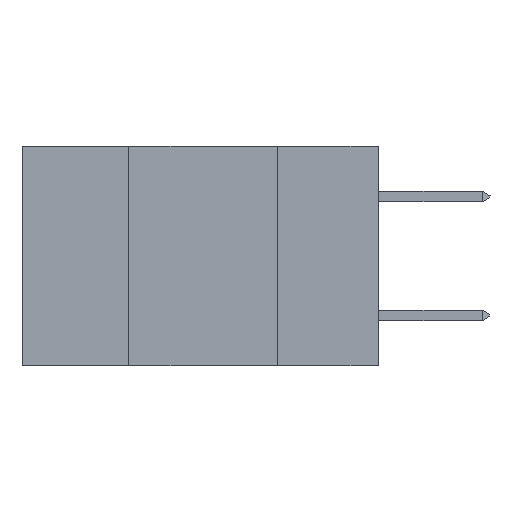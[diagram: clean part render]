
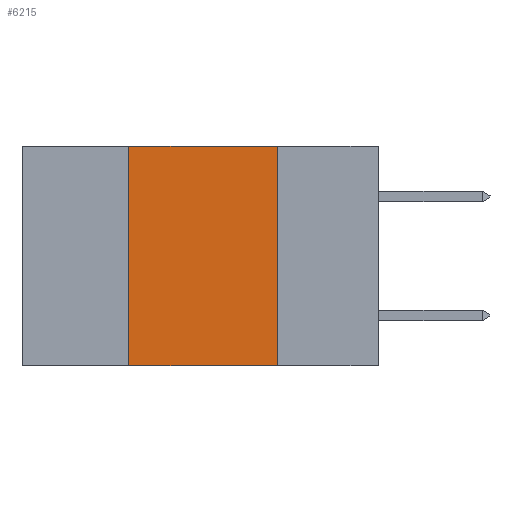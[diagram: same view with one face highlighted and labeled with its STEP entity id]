
A CAD part, left-side view. The second image highlights one B-rep face of the part: STEP entity #6215.
In plain terms, the highlighted planar face has unit normal (-1, 0, 0).
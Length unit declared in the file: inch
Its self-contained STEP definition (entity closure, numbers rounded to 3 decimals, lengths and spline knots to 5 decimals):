
#17 = CARTESIAN_POINT ( 'NONE',  ( 0., 0.6, -0.37 ) ) ;
#450 = VERTEX_POINT ( 'NONE', #5903 ) ;
#651 = ORIENTED_EDGE ( 'NONE', *, *, #9462, .T. ) ;
#883 = DIRECTION ( 'NONE',  ( 0., 0., 1. ) ) ;
#1632 = FACE_OUTER_BOUND ( 'NONE', #2516, .T. ) ;
#1798 = VECTOR ( 'NONE', #7610, 39.37008 ) ;
#2282 = VERTEX_POINT ( 'NONE', #5135 ) ;
#2516 = EDGE_LOOP ( 'NONE', ( #6229, #13106, #4326, #651 ) ) ;
#2710 = CARTESIAN_POINT ( 'NONE',  ( 0., 0.6, 0. ) ) ;
#3180 = EDGE_CURVE ( 'NONE', #2282, #3736, #10170, .T. ) ;
#3325 = CARTESIAN_POINT ( 'NONE',  ( 0., 0.17, -0.37 ) ) ;
#3348 = LINE ( 'NONE', #17, #13123 ) ;
#3736 = VERTEX_POINT ( 'NONE', #13234 ) ;
#4326 = ORIENTED_EDGE ( 'NONE', *, *, #3180, .F. ) ;
#5135 = CARTESIAN_POINT ( 'NONE',  ( 0., 0.42, -0.37 ) ) ;
#5166 = CARTESIAN_POINT ( 'NONE',  ( 0., 0.42, -0.37 ) ) ;
#5258 = DIRECTION ( 'NONE',  ( 0., -1., 0. ) ) ;
#5530 = EDGE_CURVE ( 'NONE', #3736, #450, #13012, .T. ) ;
#5903 = CARTESIAN_POINT ( 'NONE',  ( 0., 0.17, 0. ) ) ;
#6215 = ADVANCED_FACE ( 'NONE', ( #1632 ), #13239, .F. ) ;
#6229 = ORIENTED_EDGE ( 'NONE', *, *, #6527, .F. ) ;
#6527 = EDGE_CURVE ( 'NONE', #450, #10718, #7678, .T. ) ;
#7010 = DIRECTION ( 'NONE',  ( 0., 0., -1. ) ) ;
#7610 = DIRECTION ( 'NONE',  ( 0., 0., -1. ) ) ;
#7678 = LINE ( 'NONE', #3325, #1798 ) ;
#7688 = VECTOR ( 'NONE', #11098, 39.37008 ) ;
#8000 = CARTESIAN_POINT ( 'NONE',  ( 0., 0.17, -0.37 ) ) ;
#8089 = DIRECTION ( 'NONE',  ( 1., 0., 0. ) ) ;
#9462 = EDGE_CURVE ( 'NONE', #2282, #10718, #3348, .T. ) ;
#9577 = AXIS2_PLACEMENT_3D ( 'NONE', #10984, #8089, #7010 ) ;
#10170 = LINE ( 'NONE', #5166, #11445 ) ;
#10718 = VERTEX_POINT ( 'NONE', #8000 ) ;
#10984 = CARTESIAN_POINT ( 'NONE',  ( 0., 0.6, 0. ) ) ;
#11098 = DIRECTION ( 'NONE',  ( 0., -1., 0. ) ) ;
#11445 = VECTOR ( 'NONE', #883, 39.37008 ) ;
#13012 = LINE ( 'NONE', #2710, #7688 ) ;
#13106 = ORIENTED_EDGE ( 'NONE', *, *, #5530, .F. ) ;
#13123 = VECTOR ( 'NONE', #5258, 39.37008 ) ;
#13234 = CARTESIAN_POINT ( 'NONE',  ( 0., 0.42, 0. ) ) ;
#13239 = PLANE ( 'NONE',  #9577 ) ;
